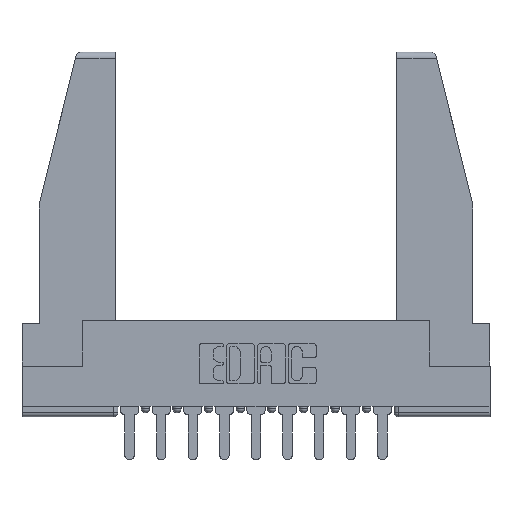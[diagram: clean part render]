
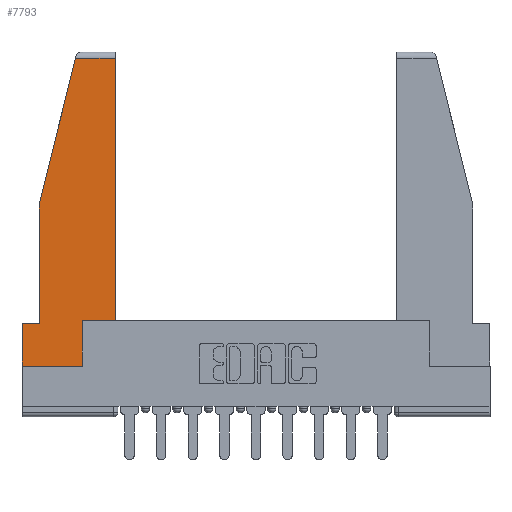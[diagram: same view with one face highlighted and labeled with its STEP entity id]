
A CAD part, top view. The second image highlights one B-rep face of the part: STEP entity #7793.
In plain terms, the highlighted planar face has unit normal (0, 0, 1).
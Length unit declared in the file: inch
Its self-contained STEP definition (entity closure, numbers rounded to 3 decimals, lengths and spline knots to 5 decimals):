
#20 = VERTEX_POINT ( 'NONE', #2912 ) ;
#111 = CARTESIAN_POINT ( 'NONE',  ( 0.461, 1.52, 0. ) ) ;
#151 = CARTESIAN_POINT ( 'NONE',  ( 0.086, 0.21, 0. ) ) ;
#367 = DIRECTION ( 'NONE',  ( -1., 0., 0. ) ) ;
#372 = VECTOR ( 'NONE', #3775, 39.37008 ) ;
#378 = ORIENTED_EDGE ( 'NONE', *, *, #4245, .T. ) ;
#539 = FACE_OUTER_BOUND ( 'NONE', #6869, .T. ) ;
#717 = AXIS2_PLACEMENT_3D ( 'NONE', #13414, #11349, #1407 ) ;
#1053 = LINE ( 'NONE', #2690, #372 ) ;
#1182 = VERTEX_POINT ( 'NONE', #111 ) ;
#1268 = CARTESIAN_POINT ( 'NONE',  ( 0., 1.52, 0. ) ) ;
#1305 = EDGE_CURVE ( 'NONE', #8956, #13148, #8469, .T. ) ;
#1407 = DIRECTION ( 'NONE',  ( 1., 0., 0. ) ) ;
#1487 = ORIENTED_EDGE ( 'NONE', *, *, #1305, .T. ) ;
#1823 = VECTOR ( 'NONE', #5980, 39.37008 ) ;
#1904 = CARTESIAN_POINT ( 'NONE',  ( 0., 0., 0. ) ) ;
#2036 = ORIENTED_EDGE ( 'NONE', *, *, #7994, .T. ) ;
#2125 = CARTESIAN_POINT ( 'NONE',  ( 0., 0., 0. ) ) ;
#2304 = DIRECTION ( 'NONE',  ( 0., 1., 0. ) ) ;
#2690 = CARTESIAN_POINT ( 'NONE',  ( 0.297, 0.223, 0. ) ) ;
#2802 = ORIENTED_EDGE ( 'NONE', *, *, #10264, .T. ) ;
#2912 = CARTESIAN_POINT ( 'NONE',  ( 0.297, 0.223, 0. ) ) ;
#3766 = CARTESIAN_POINT ( 'NONE',  ( 0.086, 0.8, 0. ) ) ;
#3775 = DIRECTION ( 'NONE',  ( 1., 0., 0. ) ) ;
#4245 = EDGE_CURVE ( 'NONE', #10987, #10707, #8899, .T. ) ;
#4381 = CARTESIAN_POINT ( 'NONE',  ( 0.461, 0.223, 0. ) ) ;
#4529 = ORIENTED_EDGE ( 'NONE', *, *, #5575, .T. ) ;
#4879 = CARTESIAN_POINT ( 'NONE',  ( 0.461, 0.223, 0. ) ) ;
#4936 = CARTESIAN_POINT ( 'NONE',  ( 0., 0.21, 0. ) ) ;
#5366 = LINE ( 'NONE', #12305, #7925 ) ;
#5395 = VECTOR ( 'NONE', #12614, 39.37008 ) ;
#5575 = EDGE_CURVE ( 'NONE', #14063, #11813, #12115, .T. ) ;
#5796 = CARTESIAN_POINT ( 'NONE',  ( 0.086, 0.8, 0. ) ) ;
#5980 = DIRECTION ( 'NONE',  ( 0., -1., 0. ) ) ;
#6713 = DIRECTION ( 'NONE',  ( 0., 1., 0. ) ) ;
#6747 = CARTESIAN_POINT ( 'NONE',  ( 0., 0.21, 0. ) ) ;
#6769 = EDGE_CURVE ( 'NONE', #10707, #20, #5366, .T. ) ;
#6801 = LINE ( 'NONE', #4381, #14204 ) ;
#6869 = EDGE_LOOP ( 'NONE', ( #11679, #6946, #4529, #2802, #1487, #9831, #378, #11873, #2036 ) ) ;
#6946 = ORIENTED_EDGE ( 'NONE', *, *, #9723, .T. ) ;
#6958 = DIRECTION ( 'NONE',  ( -0.239, -0.971, 0. ) ) ;
#6976 = LINE ( 'NONE', #3766, #1823 ) ;
#7145 = VECTOR ( 'NONE', #10143, 39.37008 ) ;
#7793 = ADVANCED_FACE ( 'NONE', ( #539 ), #7958, .T. ) ;
#7925 = VECTOR ( 'NONE', #2304, 39.37008 ) ;
#7958 = PLANE ( 'NONE',  #717 ) ;
#7994 = EDGE_CURVE ( 'NONE', #20, #12011, #1053, .T. ) ;
#8469 = LINE ( 'NONE', #11390, #13298 ) ;
#8899 = LINE ( 'NONE', #2125, #10798 ) ;
#8956 = VERTEX_POINT ( 'NONE', #151 ) ;
#8987 = LINE ( 'NONE', #4936, #5395 ) ;
#9134 = CARTESIAN_POINT ( 'NONE',  ( 0.297, 0., 0. ) ) ;
#9147 = VECTOR ( 'NONE', #6958, 39.37008 ) ;
#9303 = CARTESIAN_POINT ( 'NONE',  ( 0.2636, 1.52, 0. ) ) ;
#9723 = EDGE_CURVE ( 'NONE', #1182, #14063, #13517, .T. ) ;
#9798 = DIRECTION ( 'NONE',  ( 1., 0., 0. ) ) ;
#9831 = ORIENTED_EDGE ( 'NONE', *, *, #12018, .T. ) ;
#9940 = EDGE_CURVE ( 'NONE', #12011, #1182, #6801, .T. ) ;
#10143 = DIRECTION ( 'NONE',  ( -1., 0., 0. ) ) ;
#10264 = EDGE_CURVE ( 'NONE', #11813, #8956, #6976, .T. ) ;
#10707 = VERTEX_POINT ( 'NONE', #9134 ) ;
#10798 = VECTOR ( 'NONE', #9798, 39.37008 ) ;
#10987 = VERTEX_POINT ( 'NONE', #1904 ) ;
#11349 = DIRECTION ( 'NONE',  ( 0., 0., 1. ) ) ;
#11390 = CARTESIAN_POINT ( 'NONE',  ( 0., 0.21, 0. ) ) ;
#11679 = ORIENTED_EDGE ( 'NONE', *, *, #9940, .T. ) ;
#11813 = VERTEX_POINT ( 'NONE', #5796 ) ;
#11873 = ORIENTED_EDGE ( 'NONE', *, *, #6769, .T. ) ;
#12011 = VERTEX_POINT ( 'NONE', #4879 ) ;
#12018 = EDGE_CURVE ( 'NONE', #13148, #10987, #8987, .T. ) ;
#12115 = LINE ( 'NONE', #13595, #9147 ) ;
#12305 = CARTESIAN_POINT ( 'NONE',  ( 0.297, 0., 0. ) ) ;
#12614 = DIRECTION ( 'NONE',  ( 0., -1., 0. ) ) ;
#13148 = VERTEX_POINT ( 'NONE', #6747 ) ;
#13298 = VECTOR ( 'NONE', #367, 39.37008 ) ;
#13414 = CARTESIAN_POINT ( 'NONE',  ( 0., 0., 0. ) ) ;
#13517 = LINE ( 'NONE', #1268, #7145 ) ;
#13595 = CARTESIAN_POINT ( 'NONE',  ( 0.271, 1.55, 0. ) ) ;
#14063 = VERTEX_POINT ( 'NONE', #9303 ) ;
#14204 = VECTOR ( 'NONE', #6713, 39.37008 ) ;
